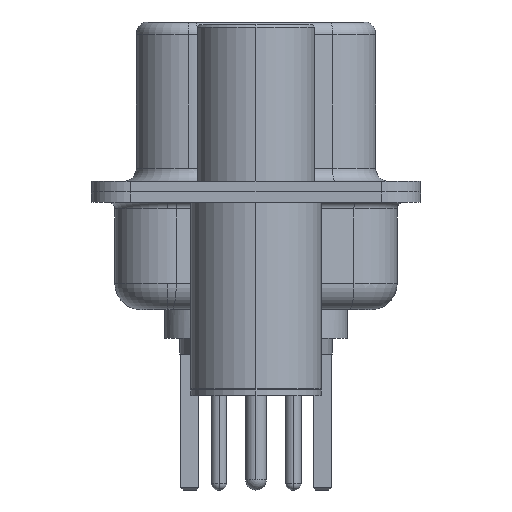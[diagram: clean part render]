
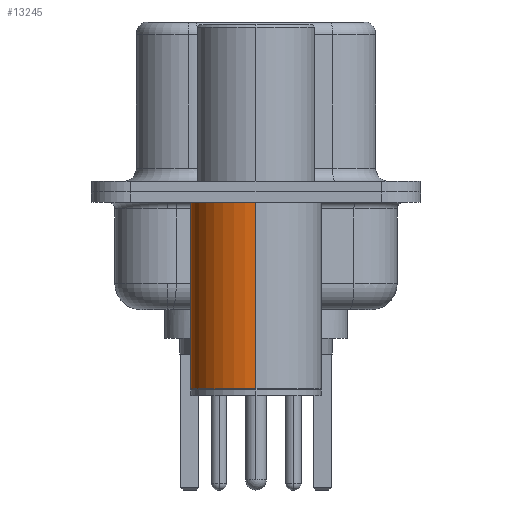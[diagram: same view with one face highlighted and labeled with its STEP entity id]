
A CAD part, left-side view. The second image highlights one B-rep face of the part: STEP entity #13245.
In plain terms, the highlighted cylindrical face has radius 2.5 mm (diameter 5 mm), a partial arc.
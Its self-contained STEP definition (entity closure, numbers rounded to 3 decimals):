
#1475 = DIRECTION ( 'NONE',  ( 0., 0., 1. ) ) ;
#1564 = DIRECTION ( 'NONE',  ( 0., 0., 1. ) ) ;
#2033 = VERTEX_POINT ( 'NONE', #16383 ) ;
#2361 = ORIENTED_EDGE ( 'NONE', *, *, #11601, .T. ) ;
#5196 = ORIENTED_EDGE ( 'NONE', *, *, #9331, .F. ) ;
#6587 = AXIS2_PLACEMENT_3D ( 'NONE', #9189, #22876, #13174 ) ;
#7428 = AXIS2_PLACEMENT_3D ( 'NONE', #22901, #11371, #24770 ) ;
#8145 = LINE ( 'NONE', #22846, #17868 ) ;
#8299 = VERTEX_POINT ( 'NONE', #22852 ) ;
#9189 = CARTESIAN_POINT ( 'NONE',  ( 0., 0., 0.581 ) ) ;
#9331 = EDGE_CURVE ( 'NONE', #21827, #8299, #13129, .T. ) ;
#9912 = EDGE_CURVE ( 'NONE', #2033, #16929, #8145, .T. ) ;
#11371 = DIRECTION ( 'NONE',  ( 0., 0., 1. ) ) ;
#11567 = EDGE_CURVE ( 'NONE', #8299, #16929, #20953, .T. ) ;
#11601 = EDGE_CURVE ( 'NONE', #21827, #2033, #19707, .T. ) ;
#12725 = EDGE_LOOP ( 'NONE', ( #2361, #23778, #22310, #5196 ) ) ;
#13129 = LINE ( 'NONE', #23045, #22786 ) ;
#13174 = DIRECTION ( 'NONE',  ( 1., 0., 0. ) ) ;
#13245 = ADVANCED_FACE ( 'NONE', ( #14571 ), #19114, .T. ) ;
#13366 = CARTESIAN_POINT ( 'NONE',  ( 0., 0., -7.525 ) ) ;
#14011 = AXIS2_PLACEMENT_3D ( 'NONE', #13366, #1475, #15263 ) ;
#14571 = FACE_OUTER_BOUND ( 'NONE', #12725, .T. ) ;
#15263 = DIRECTION ( 'NONE',  ( 1., 0., 0. ) ) ;
#16383 = CARTESIAN_POINT ( 'NONE',  ( -2.5, 0., -7.525 ) ) ;
#16929 = VERTEX_POINT ( 'NONE', #17629 ) ;
#17099 = CARTESIAN_POINT ( 'NONE',  ( 2.5, 0., -7.525 ) ) ;
#17629 = CARTESIAN_POINT ( 'NONE',  ( -2.5, 0., -0.4 ) ) ;
#17868 = VECTOR ( 'NONE', #18946, 1000. ) ;
#18946 = DIRECTION ( 'NONE',  ( 0., 0., 1. ) ) ;
#19114 = CYLINDRICAL_SURFACE ( 'NONE', #6587, 2.5 ) ;
#19707 = CIRCLE ( 'NONE', #14011, 2.5 ) ;
#20953 = CIRCLE ( 'NONE', #7428, 2.5 ) ;
#21827 = VERTEX_POINT ( 'NONE', #17099 ) ;
#22310 = ORIENTED_EDGE ( 'NONE', *, *, #11567, .F. ) ;
#22786 = VECTOR ( 'NONE', #1564, 1000. ) ;
#22846 = CARTESIAN_POINT ( 'NONE',  ( -2.5, 0., 0.581 ) ) ;
#22852 = CARTESIAN_POINT ( 'NONE',  ( 2.5, 0., -0.4 ) ) ;
#22876 = DIRECTION ( 'NONE',  ( 0., 0., 1. ) ) ;
#22901 = CARTESIAN_POINT ( 'NONE',  ( 0., 0., -0.4 ) ) ;
#23045 = CARTESIAN_POINT ( 'NONE',  ( 2.5, 0., 0.581 ) ) ;
#23778 = ORIENTED_EDGE ( 'NONE', *, *, #9912, .T. ) ;
#24770 = DIRECTION ( 'NONE',  ( 1., 0., 0. ) ) ;
